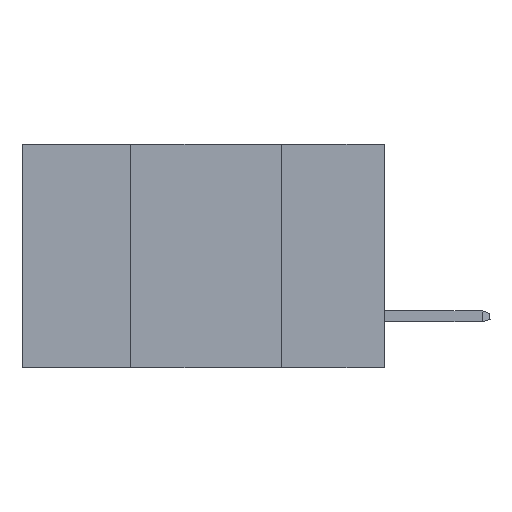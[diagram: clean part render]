
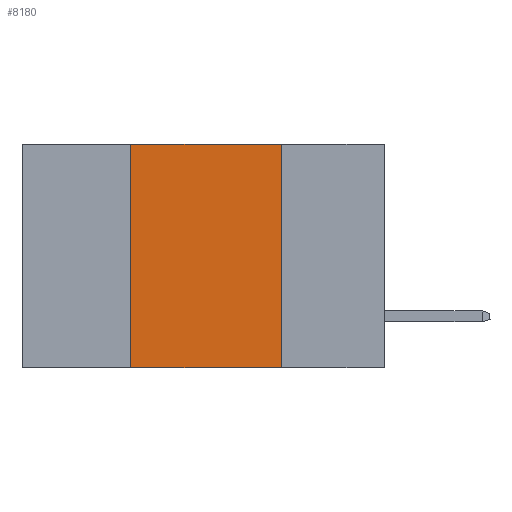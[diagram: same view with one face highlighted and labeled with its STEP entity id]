
A CAD part, left-side view. The second image highlights one B-rep face of the part: STEP entity #8180.
In plain terms, the highlighted planar face has unit normal (-1, 0, 0).
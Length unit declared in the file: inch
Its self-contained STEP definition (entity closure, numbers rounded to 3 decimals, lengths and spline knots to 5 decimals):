
#955 = DIRECTION ( 'NONE',  ( 0., 0., 1. ) ) ;
#1226 = CARTESIAN_POINT ( 'NONE',  ( 0., 0.42, -0.37 ) ) ;
#2350 = EDGE_CURVE ( 'NONE', #8526, #7209, #7688, .T. ) ;
#2543 = DIRECTION ( 'NONE',  ( 0., -1., 0. ) ) ;
#3230 = ORIENTED_EDGE ( 'NONE', *, *, #2350, .F. ) ;
#3607 = ORIENTED_EDGE ( 'NONE', *, *, #14905, .F. ) ;
#3695 = VECTOR ( 'NONE', #22287, 39.37008 ) ;
#4316 = LINE ( 'NONE', #14718, #3695 ) ;
#5005 = LINE ( 'NONE', #8511, #14165 ) ;
#5398 = CARTESIAN_POINT ( 'NONE',  ( 0., 0.17, 0. ) ) ;
#6983 = DIRECTION ( 'NONE',  ( 1., 0., 0. ) ) ;
#7209 = VERTEX_POINT ( 'NONE', #21200 ) ;
#7688 = LINE ( 'NONE', #16895, #20531 ) ;
#8180 = ADVANCED_FACE ( 'NONE', ( #18741 ), #13159, .F. ) ;
#8497 = VERTEX_POINT ( 'NONE', #13139 ) ;
#8511 = CARTESIAN_POINT ( 'NONE',  ( 0., 0.6, 0. ) ) ;
#8526 = VERTEX_POINT ( 'NONE', #1226 ) ;
#9752 = VERTEX_POINT ( 'NONE', #5398 ) ;
#13139 = CARTESIAN_POINT ( 'NONE',  ( 0., 0.17, -0.37 ) ) ;
#13159 = PLANE ( 'NONE',  #16448 ) ;
#14165 = VECTOR ( 'NONE', #2543, 39.37008 ) ;
#14718 = CARTESIAN_POINT ( 'NONE',  ( 0., 0.6, -0.37 ) ) ;
#14888 = CARTESIAN_POINT ( 'NONE',  ( 0., 0.17, 0. ) ) ;
#14905 = EDGE_CURVE ( 'NONE', #7209, #9752, #5005, .T. ) ;
#15010 = CARTESIAN_POINT ( 'NONE',  ( 0., 0.6, 0. ) ) ;
#15787 = EDGE_LOOP ( 'NONE', ( #23470, #3607, #3230, #16322 ) ) ;
#16322 = ORIENTED_EDGE ( 'NONE', *, *, #20776, .T. ) ;
#16448 = AXIS2_PLACEMENT_3D ( 'NONE', #15010, #6983, #16831 ) ;
#16831 = DIRECTION ( 'NONE',  ( 0., 0., -1. ) ) ;
#16895 = CARTESIAN_POINT ( 'NONE',  ( 0., 0.42, 0. ) ) ;
#18741 = FACE_OUTER_BOUND ( 'NONE', #15787, .T. ) ;
#20531 = VECTOR ( 'NONE', #955, 39.37008 ) ;
#20776 = EDGE_CURVE ( 'NONE', #8526, #8497, #4316, .T. ) ;
#21200 = CARTESIAN_POINT ( 'NONE',  ( 0., 0.42, 0. ) ) ;
#21245 = LINE ( 'NONE', #14888, #22153 ) ;
#22153 = VECTOR ( 'NONE', #24736, 39.37008 ) ;
#22287 = DIRECTION ( 'NONE',  ( 0., -1., 0. ) ) ;
#23470 = ORIENTED_EDGE ( 'NONE', *, *, #24389, .F. ) ;
#24389 = EDGE_CURVE ( 'NONE', #9752, #8497, #21245, .T. ) ;
#24736 = DIRECTION ( 'NONE',  ( 0., 0., -1. ) ) ;
